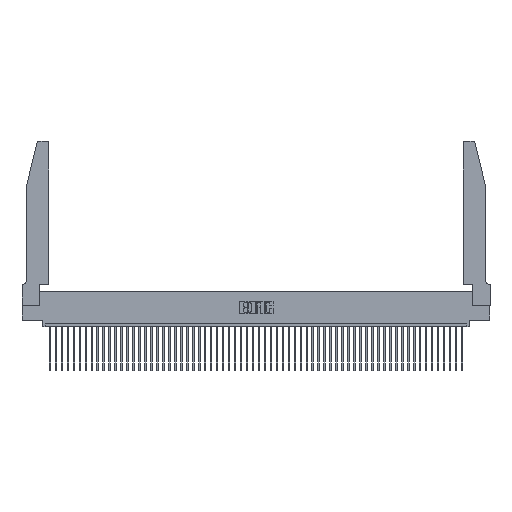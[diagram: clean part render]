
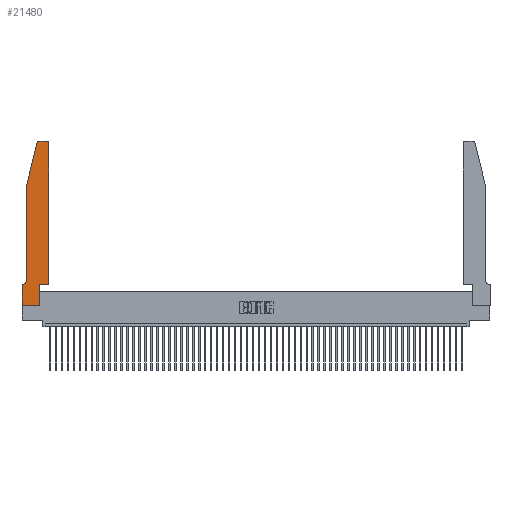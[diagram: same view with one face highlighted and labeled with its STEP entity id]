
A CAD part, top view. The second image highlights one B-rep face of the part: STEP entity #21480.
In plain terms, the highlighted planar face has unit normal (0, 0, 1).
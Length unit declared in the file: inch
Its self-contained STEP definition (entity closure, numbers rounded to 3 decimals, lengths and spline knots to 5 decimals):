
#583 = DIRECTION ( 'NONE',  ( 1., 0., 0. ) ) ;
#639 = CARTESIAN_POINT ( 'NONE',  ( 0., 0., 0.37 ) ) ;
#1059 = VECTOR ( 'NONE', #15178, 39.37008 ) ;
#1176 = LINE ( 'NONE', #46893, #31739 ) ;
#1690 = VERTEX_POINT ( 'NONE', #37195 ) ;
#1717 = DIRECTION ( 'NONE',  ( 1., 0., 0. ) ) ;
#1742 = VERTEX_POINT ( 'NONE', #17963 ) ;
#2516 = DIRECTION ( 'NONE',  ( 0., 0., -1. ) ) ;
#2662 = VECTOR ( 'NONE', #1717, 39.37008 ) ;
#3204 = CARTESIAN_POINT ( 'NONE',  ( 0.4205, 2.75, 0.37 ) ) ;
#3239 = EDGE_CURVE ( 'NONE', #11183, #47240, #25335, .T. ) ;
#4254 = CARTESIAN_POINT ( 'NONE',  ( 0., 0.35, 0.37 ) ) ;
#4499 = CARTESIAN_POINT ( 'NONE',  ( 0.4205, 2.72, 0.37 ) ) ;
#4632 = LINE ( 'NONE', #51644, #37799 ) ;
#4756 = DIRECTION ( 'NONE',  ( 0., 0., 1. ) ) ;
#5223 = VECTOR ( 'NONE', #20944, 39.37008 ) ;
#5339 = ORIENTED_EDGE ( 'NONE', *, *, #39478, .T. ) ;
#5648 = CARTESIAN_POINT ( 'NONE',  ( 0.4505, 0.35, 0.37 ) ) ;
#5884 = VERTEX_POINT ( 'NONE', #18167 ) ;
#6561 = DIRECTION ( 'NONE',  ( 0., -1., 0. ) ) ;
#6572 = AXIS2_PLACEMENT_3D ( 'NONE', #50334, #30105, #583 ) ;
#7379 = VERTEX_POINT ( 'NONE', #19386 ) ;
#7755 = EDGE_CURVE ( 'NONE', #25476, #1742, #4632, .T. ) ;
#7948 = CARTESIAN_POINT ( 'NONE',  ( 0.4505, 2.72, 0.37 ) ) ;
#8111 = ORIENTED_EDGE ( 'NONE', *, *, #29621, .T. ) ;
#8234 = LINE ( 'NONE', #20001, #1059 ) ;
#8820 = DIRECTION ( 'NONE',  ( 1., 0., 0. ) ) ;
#9232 = AXIS2_PLACEMENT_3D ( 'NONE', #35725, #2516, #14983 ) ;
#9798 = EDGE_CURVE ( 'NONE', #47240, #41325, #42847, .T. ) ;
#9939 = ORIENTED_EDGE ( 'NONE', *, *, #23093, .T. ) ;
#11014 = VECTOR ( 'NONE', #6561, 39.37008 ) ;
#11048 = DIRECTION ( 'NONE',  ( -0.239, -0.971, 0. ) ) ;
#11183 = VERTEX_POINT ( 'NONE', #5648 ) ;
#11428 = VERTEX_POINT ( 'NONE', #48351 ) ;
#11716 = CARTESIAN_POINT ( 'NONE',  ( 0.2865, 0.35, 0.37 ) ) ;
#12046 = ORIENTED_EDGE ( 'NONE', *, *, #41027, .T. ) ;
#12691 = CARTESIAN_POINT ( 'NONE',  ( 0.2605, 2.75, 0.37 ) ) ;
#12773 = DIRECTION ( 'NONE',  ( 0., 0., 1. ) ) ;
#12976 = LINE ( 'NONE', #11716, #5223 ) ;
#14488 = CARTESIAN_POINT ( 'NONE',  ( 0.0755, 2., 0.37 ) ) ;
#14983 = DIRECTION ( 'NONE',  ( -1., 0., 0. ) ) ;
#15178 = DIRECTION ( 'NONE',  ( -1., 0., 0. ) ) ;
#16024 = ORIENTED_EDGE ( 'NONE', *, *, #3239, .T. ) ;
#17963 = CARTESIAN_POINT ( 'NONE',  ( 0.0755, 0.42, 0.37 ) ) ;
#18167 = CARTESIAN_POINT ( 'NONE',  ( 0.2865, 0.35, 0.37 ) ) ;
#18984 = FACE_OUTER_BOUND ( 'NONE', #31685, .T. ) ;
#19386 = CARTESIAN_POINT ( 'NONE',  ( 0.2865, 0., 0.37 ) ) ;
#19836 = AXIS2_PLACEMENT_3D ( 'NONE', #4254, #4756, #37995 ) ;
#20001 = CARTESIAN_POINT ( 'NONE',  ( 0.0755, 0.35, 0.37 ) ) ;
#20270 = ORIENTED_EDGE ( 'NONE', *, *, #35248, .T. ) ;
#20944 = DIRECTION ( 'NONE',  ( 0., 1., 0. ) ) ;
#21480 = ADVANCED_FACE ( 'NONE', ( #18984 ), #45869, .T. ) ;
#21930 = DIRECTION ( 'NONE',  ( 1., 0., 0. ) ) ;
#23093 = EDGE_CURVE ( 'NONE', #1690, #29635, #31121, .T. ) ;
#23420 = CIRCLE ( 'NONE', #6572, 0.03 ) ;
#24683 = AXIS2_PLACEMENT_3D ( 'NONE', #4499, #12773, #8820 ) ;
#24805 = VECTOR ( 'NONE', #42904, 39.37008 ) ;
#25335 = LINE ( 'NONE', #31078, #46207 ) ;
#25476 = VERTEX_POINT ( 'NONE', #26287 ) ;
#26287 = CARTESIAN_POINT ( 'NONE',  ( 0.0755, 2., 0.37 ) ) ;
#26714 = DIRECTION ( 'NONE',  ( 0., -1., 0. ) ) ;
#26832 = EDGE_CURVE ( 'NONE', #28814, #1690, #8234, .T. ) ;
#28579 = CARTESIAN_POINT ( 'NONE',  ( 0.0055, 0.35, 0.37 ) ) ;
#28814 = VERTEX_POINT ( 'NONE', #28579 ) ;
#28911 = ORIENTED_EDGE ( 'NONE', *, *, #7755, .T. ) ;
#29621 = EDGE_CURVE ( 'NONE', #7379, #5884, #12976, .T. ) ;
#29635 = VERTEX_POINT ( 'NONE', #639 ) ;
#29996 = EDGE_CURVE ( 'NONE', #11428, #51417, #23420, .T. ) ;
#30105 = DIRECTION ( 'NONE',  ( 0., 0., 1. ) ) ;
#31078 = CARTESIAN_POINT ( 'NONE',  ( 0.4505, 0.35, 0.37 ) ) ;
#31121 = LINE ( 'NONE', #48546, #11014 ) ;
#31685 = EDGE_LOOP ( 'NONE', ( #20270, #34260, #5339, #28911, #35262, #43781, #9939, #12046, #8111, #50225, #16024, #32700 ) ) ;
#31739 = VECTOR ( 'NONE', #21930, 39.37008 ) ;
#32700 = ORIENTED_EDGE ( 'NONE', *, *, #9798, .T. ) ;
#34260 = ORIENTED_EDGE ( 'NONE', *, *, #29996, .T. ) ;
#35025 = LINE ( 'NONE', #14488, #36460 ) ;
#35248 = EDGE_CURVE ( 'NONE', #41325, #11428, #46902, .T. ) ;
#35262 = ORIENTED_EDGE ( 'NONE', *, *, #52780, .T. ) ;
#35725 = CARTESIAN_POINT ( 'NONE',  ( 0.0055, 0.42, 0.37 ) ) ;
#36416 = CARTESIAN_POINT ( 'NONE',  ( 0.25487, 2.72718, 0.37 ) ) ;
#36460 = VECTOR ( 'NONE', #11048, 39.37008 ) ;
#37195 = CARTESIAN_POINT ( 'NONE',  ( 0., 0.35, 0.37 ) ) ;
#37799 = VECTOR ( 'NONE', #26714, 39.37008 ) ;
#37995 = DIRECTION ( 'NONE',  ( 1., 0., 0. ) ) ;
#38481 = DIRECTION ( 'NONE',  ( 0., 1., 0. ) ) ;
#39478 = EDGE_CURVE ( 'NONE', #51417, #25476, #35025, .T. ) ;
#40067 = EDGE_CURVE ( 'NONE', #5884, #11183, #50001, .T. ) ;
#41027 = EDGE_CURVE ( 'NONE', #29635, #7379, #1176, .T. ) ;
#41325 = VERTEX_POINT ( 'NONE', #3204 ) ;
#42847 = CIRCLE ( 'NONE', #24683, 0.03 ) ;
#42904 = DIRECTION ( 'NONE',  ( -1., 0., 0. ) ) ;
#43781 = ORIENTED_EDGE ( 'NONE', *, *, #26832, .T. ) ;
#45869 = PLANE ( 'NONE',  #19836 ) ;
#46207 = VECTOR ( 'NONE', #38481, 39.37008 ) ;
#46893 = CARTESIAN_POINT ( 'NONE',  ( 0., 0., 0.37 ) ) ;
#46902 = LINE ( 'NONE', #12691, #24805 ) ;
#46927 = CARTESIAN_POINT ( 'NONE',  ( 0.4505, 0.35, 0.37 ) ) ;
#47240 = VERTEX_POINT ( 'NONE', #7948 ) ;
#48351 = CARTESIAN_POINT ( 'NONE',  ( 0.284, 2.75, 0.37 ) ) ;
#48546 = CARTESIAN_POINT ( 'NONE',  ( 0., 0., 0.37 ) ) ;
#50001 = LINE ( 'NONE', #46927, #2662 ) ;
#50225 = ORIENTED_EDGE ( 'NONE', *, *, #40067, .T. ) ;
#50334 = CARTESIAN_POINT ( 'NONE',  ( 0.284, 2.72, 0.37 ) ) ;
#51417 = VERTEX_POINT ( 'NONE', #36416 ) ;
#51644 = CARTESIAN_POINT ( 'NONE',  ( 0.0755, 2., 0.37 ) ) ;
#52780 = EDGE_CURVE ( 'NONE', #1742, #28814, #53724, .T. ) ;
#53724 = CIRCLE ( 'NONE', #9232, 0.07 ) ;
